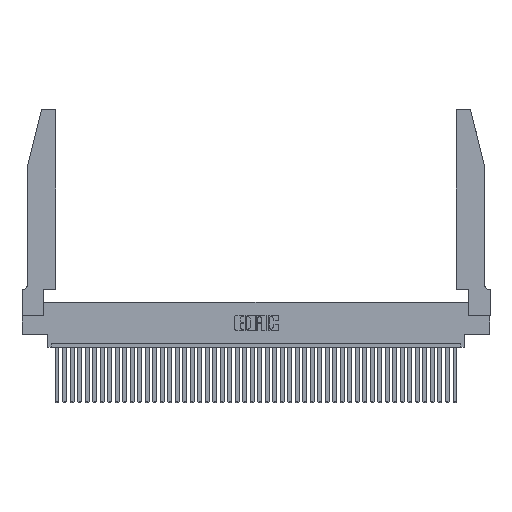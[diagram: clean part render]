
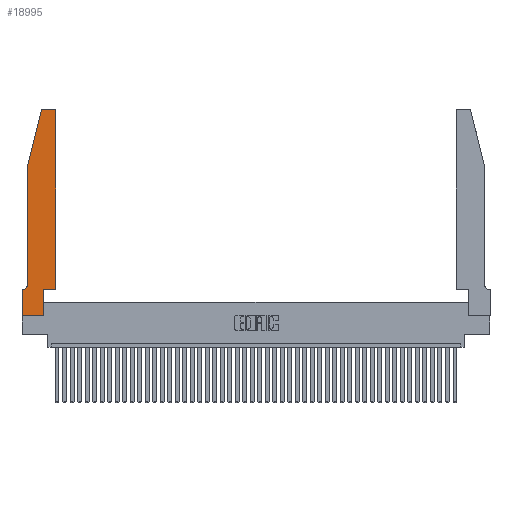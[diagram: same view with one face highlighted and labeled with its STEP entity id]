
A CAD part, top view. The second image highlights one B-rep face of the part: STEP entity #18995.
In plain terms, the highlighted planar face has unit normal (0, 0, 1).
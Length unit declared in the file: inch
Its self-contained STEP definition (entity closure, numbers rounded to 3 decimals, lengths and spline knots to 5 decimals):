
#321 = VECTOR ( 'NONE', #9406, 39.37008 ) ;
#2312 = ORIENTED_EDGE ( 'NONE', *, *, #43476, .T. ) ;
#2477 = DIRECTION ( 'NONE',  ( 1., 0., 0. ) ) ;
#2950 = DIRECTION ( 'NONE',  ( 0., -1., 0. ) ) ;
#2957 = EDGE_CURVE ( 'NONE', #3370, #42501, #36275, .T. ) ;
#3071 = VERTEX_POINT ( 'NONE', #26094 ) ;
#3219 = CARTESIAN_POINT ( 'NONE',  ( 0.4205, 2.75, 0.37 ) ) ;
#3370 = VERTEX_POINT ( 'NONE', #24207 ) ;
#3528 = ORIENTED_EDGE ( 'NONE', *, *, #39420, .T. ) ;
#3818 = VECTOR ( 'NONE', #29422, 39.37008 ) ;
#4001 = CIRCLE ( 'NONE', #30791, 0.03 ) ;
#4253 = CARTESIAN_POINT ( 'NONE',  ( 0., 0., 0.37 ) ) ;
#4394 = DIRECTION ( 'NONE',  ( 0., 0., -1. ) ) ;
#5098 = EDGE_CURVE ( 'NONE', #37621, #25265, #21299, .T. ) ;
#5205 = ORIENTED_EDGE ( 'NONE', *, *, #9554, .T. ) ;
#5430 = ORIENTED_EDGE ( 'NONE', *, *, #23299, .T. ) ;
#5642 = EDGE_CURVE ( 'NONE', #6585, #37621, #34922, .T. ) ;
#5746 = DIRECTION ( 'NONE',  ( 0., 0., 1. ) ) ;
#5863 = AXIS2_PLACEMENT_3D ( 'NONE', #21438, #4394, #17621 ) ;
#5945 = DIRECTION ( 'NONE',  ( 0., 0., 1. ) ) ;
#6440 = VECTOR ( 'NONE', #24730, 39.37008 ) ;
#6585 = VERTEX_POINT ( 'NONE', #9338 ) ;
#7117 = CARTESIAN_POINT ( 'NONE',  ( 0.0755, 0.35, 0.37 ) ) ;
#7452 = VERTEX_POINT ( 'NONE', #42268 ) ;
#7900 = EDGE_CURVE ( 'NONE', #20560, #13302, #8405, .T. ) ;
#8203 = LINE ( 'NONE', #31666, #25155 ) ;
#8405 = LINE ( 'NONE', #43178, #10999 ) ;
#8897 = AXIS2_PLACEMENT_3D ( 'NONE', #12120, #5945, #39284 ) ;
#9256 = CARTESIAN_POINT ( 'NONE',  ( 0.0755, 2., 0.37 ) ) ;
#9338 = CARTESIAN_POINT ( 'NONE',  ( 0.4505, 0.35, 0.37 ) ) ;
#9406 = DIRECTION ( 'NONE',  ( -0.239, -0.971, 0. ) ) ;
#9554 = EDGE_CURVE ( 'NONE', #3071, #6585, #32696, .T. ) ;
#9557 = DIRECTION ( 'NONE',  ( 1., 0., 0. ) ) ;
#10343 = FACE_OUTER_BOUND ( 'NONE', #12545, .T. ) ;
#10585 = CARTESIAN_POINT ( 'NONE',  ( 0.4505, 0.35, 0.37 ) ) ;
#10999 = VECTOR ( 'NONE', #9557, 39.37008 ) ;
#11254 = ORIENTED_EDGE ( 'NONE', *, *, #2957, .T. ) ;
#11369 = VECTOR ( 'NONE', #13582, 39.37008 ) ;
#11647 = ORIENTED_EDGE ( 'NONE', *, *, #35200, .T. ) ;
#11790 = AXIS2_PLACEMENT_3D ( 'NONE', #22612, #5746, #2477 ) ;
#12120 = CARTESIAN_POINT ( 'NONE',  ( 0.4205, 2.72, 0.37 ) ) ;
#12545 = EDGE_LOOP ( 'NONE', ( #15407, #38773, #11254, #2312, #3528, #26665, #11647, #17398, #5430, #5205, #14714, #19375 ) ) ;
#12580 = VERTEX_POINT ( 'NONE', #38575 ) ;
#13302 = VERTEX_POINT ( 'NONE', #27398 ) ;
#13338 = CIRCLE ( 'NONE', #5863, 0.07 ) ;
#13582 = DIRECTION ( 'NONE',  ( 0., -1., 0. ) ) ;
#14714 = ORIENTED_EDGE ( 'NONE', *, *, #5642, .T. ) ;
#14875 = VECTOR ( 'NONE', #40950, 39.37008 ) ;
#15407 = ORIENTED_EDGE ( 'NONE', *, *, #28971, .T. ) ;
#15759 = CARTESIAN_POINT ( 'NONE',  ( 0.0755, 2., 0.37 ) ) ;
#16012 = CARTESIAN_POINT ( 'NONE',  ( 0.284, 2.72, 0.37 ) ) ;
#17398 = ORIENTED_EDGE ( 'NONE', *, *, #7900, .T. ) ;
#17621 = DIRECTION ( 'NONE',  ( -1., 0., 0. ) ) ;
#18544 = EDGE_CURVE ( 'NONE', #43497, #3370, #4001, .T. ) ;
#18995 = ADVANCED_FACE ( 'NONE', ( #10343 ), #35677, .T. ) ;
#19375 = ORIENTED_EDGE ( 'NONE', *, *, #5098, .T. ) ;
#19707 = CARTESIAN_POINT ( 'NONE',  ( 0.0055, 0.35, 0.37 ) ) ;
#20133 = CARTESIAN_POINT ( 'NONE',  ( 0.284, 2.75, 0.37 ) ) ;
#20560 = VERTEX_POINT ( 'NONE', #4253 ) ;
#21299 = CIRCLE ( 'NONE', #8897, 0.03 ) ;
#21438 = CARTESIAN_POINT ( 'NONE',  ( 0.0055, 0.42, 0.37 ) ) ;
#22274 = LINE ( 'NONE', #41894, #6440 ) ;
#22612 = CARTESIAN_POINT ( 'NONE',  ( 0., 0.35, 0.37 ) ) ;
#22826 = DIRECTION ( 'NONE',  ( 1., 0., 0. ) ) ;
#23299 = EDGE_CURVE ( 'NONE', #13302, #3071, #8203, .T. ) ;
#23782 = VECTOR ( 'NONE', #33005, 39.37008 ) ;
#24207 = CARTESIAN_POINT ( 'NONE',  ( 0.25487, 2.72718, 0.37 ) ) ;
#24730 = DIRECTION ( 'NONE',  ( -1., 0., 0. ) ) ;
#25155 = VECTOR ( 'NONE', #41225, 39.37008 ) ;
#25265 = VERTEX_POINT ( 'NONE', #3219 ) ;
#25976 = CARTESIAN_POINT ( 'NONE',  ( 0.4505, 0.35, 0.37 ) ) ;
#26094 = CARTESIAN_POINT ( 'NONE',  ( 0.2865, 0.35, 0.37 ) ) ;
#26665 = ORIENTED_EDGE ( 'NONE', *, *, #27990, .T. ) ;
#27398 = CARTESIAN_POINT ( 'NONE',  ( 0.2865, 0., 0.37 ) ) ;
#27609 = CARTESIAN_POINT ( 'NONE',  ( 0., 0., 0.37 ) ) ;
#27640 = CARTESIAN_POINT ( 'NONE',  ( 0.4505, 2.72, 0.37 ) ) ;
#27990 = EDGE_CURVE ( 'NONE', #42042, #7452, #39215, .T. ) ;
#28971 = EDGE_CURVE ( 'NONE', #25265, #43497, #22274, .T. ) ;
#29422 = DIRECTION ( 'NONE',  ( -1., 0., 0. ) ) ;
#30442 = CARTESIAN_POINT ( 'NONE',  ( 0.0755, 2., 0.37 ) ) ;
#30791 = AXIS2_PLACEMENT_3D ( 'NONE', #16012, #42976, #22826 ) ;
#31666 = CARTESIAN_POINT ( 'NONE',  ( 0.2865, 0.35, 0.37 ) ) ;
#31977 = LINE ( 'NONE', #30442, #11369 ) ;
#32696 = LINE ( 'NONE', #25976, #23782 ) ;
#33005 = DIRECTION ( 'NONE',  ( 1., 0., 0. ) ) ;
#34922 = LINE ( 'NONE', #10585, #14875 ) ;
#35200 = EDGE_CURVE ( 'NONE', #7452, #20560, #38983, .T. ) ;
#35677 = PLANE ( 'NONE',  #11790 ) ;
#36275 = LINE ( 'NONE', #9256, #321 ) ;
#37621 = VERTEX_POINT ( 'NONE', #27640 ) ;
#38575 = CARTESIAN_POINT ( 'NONE',  ( 0.0755, 0.42, 0.37 ) ) ;
#38773 = ORIENTED_EDGE ( 'NONE', *, *, #18544, .T. ) ;
#38983 = LINE ( 'NONE', #27609, #39539 ) ;
#39215 = LINE ( 'NONE', #7117, #3818 ) ;
#39284 = DIRECTION ( 'NONE',  ( 1., 0., 0. ) ) ;
#39420 = EDGE_CURVE ( 'NONE', #12580, #42042, #13338, .T. ) ;
#39539 = VECTOR ( 'NONE', #2950, 39.37008 ) ;
#40950 = DIRECTION ( 'NONE',  ( 0., 1., 0. ) ) ;
#41225 = DIRECTION ( 'NONE',  ( 0., 1., 0. ) ) ;
#41894 = CARTESIAN_POINT ( 'NONE',  ( 0.2605, 2.75, 0.37 ) ) ;
#42042 = VERTEX_POINT ( 'NONE', #19707 ) ;
#42268 = CARTESIAN_POINT ( 'NONE',  ( 0., 0.35, 0.37 ) ) ;
#42501 = VERTEX_POINT ( 'NONE', #15759 ) ;
#42976 = DIRECTION ( 'NONE',  ( 0., 0., 1. ) ) ;
#43178 = CARTESIAN_POINT ( 'NONE',  ( 0., 0., 0.37 ) ) ;
#43476 = EDGE_CURVE ( 'NONE', #42501, #12580, #31977, .T. ) ;
#43497 = VERTEX_POINT ( 'NONE', #20133 ) ;
